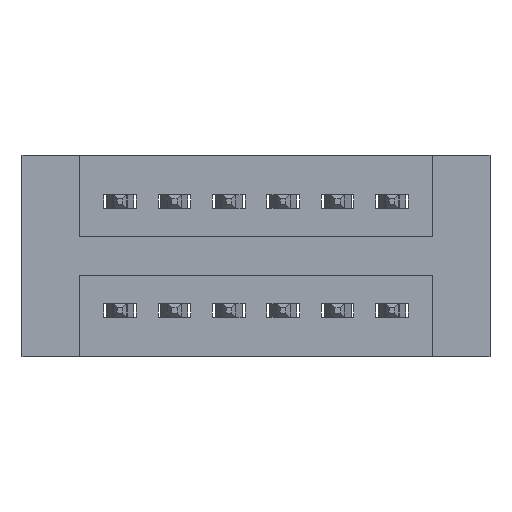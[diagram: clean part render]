
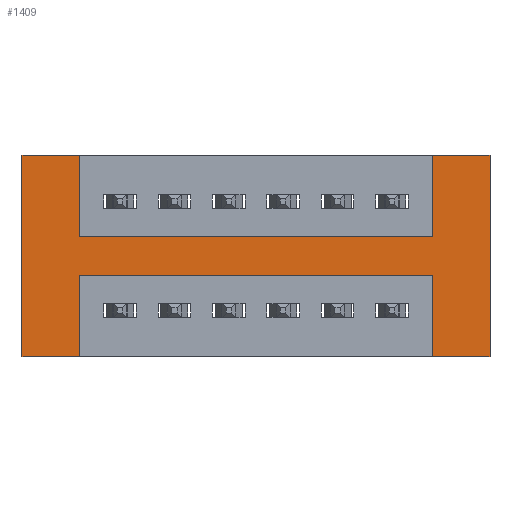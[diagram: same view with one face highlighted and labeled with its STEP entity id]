
A CAD part, front view. The second image highlights one B-rep face of the part: STEP entity #1409.
In plain terms, the highlighted planar face has unit normal (0, -1, 0).
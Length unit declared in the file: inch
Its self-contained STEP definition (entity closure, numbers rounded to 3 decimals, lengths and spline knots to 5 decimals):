
#89 = ORIENTED_EDGE ( 'NONE', *, *, #5785, .F. ) ;
#138 = CARTESIAN_POINT ( 'NONE',  ( 0.3925, 0., -0.15 ) ) ;
#204 = CARTESIAN_POINT ( 'NONE',  ( 0., 0., 0. ) ) ;
#241 = EDGE_CURVE ( 'NONE', #8746, #2887, #8727, .T. ) ;
#384 = VERTEX_POINT ( 'NONE', #6735 ) ;
#539 = VECTOR ( 'NONE', #4128, 39.37008 ) ;
#594 = VECTOR ( 'NONE', #5616, 39.37008 ) ;
#743 = PLANE ( 'NONE',  #5695 ) ;
#817 = VERTEX_POINT ( 'NONE', #7355 ) ;
#935 = EDGE_CURVE ( 'NONE', #8474, #6938, #4591, .T. ) ;
#956 = CARTESIAN_POINT ( 'NONE',  ( 0.2875, 0., 0. ) ) ;
#963 = CARTESIAN_POINT ( 'NONE',  ( 0.3925, 0., -0.15 ) ) ;
#1040 = DIRECTION ( 'NONE',  ( 0., 0., -1. ) ) ;
#1363 = VECTOR ( 'NONE', #9132, 39.37008 ) ;
#1395 = EDGE_CURVE ( 'NONE', #8628, #8474, #2612, .T. ) ;
#1409 = ADVANCED_FACE ( 'NONE', ( #6409 ), #743, .T. ) ;
#1860 = CARTESIAN_POINT ( 'NONE',  ( 0.3925, 0., 0. ) ) ;
#2245 = VERTEX_POINT ( 'NONE', #7842 ) ;
#2431 = EDGE_CURVE ( 'NONE', #5949, #2245, #8277, .T. ) ;
#2488 = LINE ( 'NONE', #2884, #6074 ) ;
#2534 = EDGE_CURVE ( 'NONE', #2245, #5627, #7633, .T. ) ;
#2536 = LINE ( 'NONE', #4183, #539 ) ;
#2612 = LINE ( 'NONE', #6999, #8086 ) ;
#2793 = VECTOR ( 'NONE', #4231, 39.37008 ) ;
#2884 = CARTESIAN_POINT ( 'NONE',  ( 0.3925, 0., -0.22 ) ) ;
#2887 = VERTEX_POINT ( 'NONE', #8492 ) ;
#2954 = CARTESIAN_POINT ( 'NONE',  ( 0.3925, 0., -0.22 ) ) ;
#3078 = LINE ( 'NONE', #4296, #6582 ) ;
#3406 = ORIENTED_EDGE ( 'NONE', *, *, #4635, .F. ) ;
#3636 = CARTESIAN_POINT ( 'NONE',  ( 1.0425, 0., -0.15 ) ) ;
#3640 = DIRECTION ( 'NONE',  ( -1., 0., 0. ) ) ;
#3722 = LINE ( 'NONE', #204, #9209 ) ;
#3738 = ORIENTED_EDGE ( 'NONE', *, *, #2534, .F. ) ;
#3787 = ORIENTED_EDGE ( 'NONE', *, *, #5757, .F. ) ;
#3859 = LINE ( 'NONE', #956, #7163 ) ;
#3908 = CARTESIAN_POINT ( 'NONE',  ( 1.0425, 0., 0. ) ) ;
#4039 = DIRECTION ( 'NONE',  ( 0., 0., 1. ) ) ;
#4128 = DIRECTION ( 'NONE',  ( 1., 0., 0. ) ) ;
#4182 = ORIENTED_EDGE ( 'NONE', *, *, #6571, .F. ) ;
#4183 = CARTESIAN_POINT ( 'NONE',  ( 0., 0., 0. ) ) ;
#4196 = CARTESIAN_POINT ( 'NONE',  ( 1.1475, 0., 0. ) ) ;
#4230 = DIRECTION ( 'NONE',  ( 0., 0., -1. ) ) ;
#4231 = DIRECTION ( 'NONE',  ( 0., 0., 1. ) ) ;
#4296 = CARTESIAN_POINT ( 'NONE',  ( 0., 0., -0.37 ) ) ;
#4338 = DIRECTION ( 'NONE',  ( -1., 0., 0. ) ) ;
#4471 = CARTESIAN_POINT ( 'NONE',  ( 0., 0., -0.37 ) ) ;
#4517 = LINE ( 'NONE', #3908, #8022 ) ;
#4591 = LINE ( 'NONE', #963, #7893 ) ;
#4635 = EDGE_CURVE ( 'NONE', #8648, #8746, #3078, .T. ) ;
#4803 = CARTESIAN_POINT ( 'NONE',  ( 0.2875, 0., -0.37 ) ) ;
#4810 = EDGE_CURVE ( 'NONE', #384, #5627, #3859, .T. ) ;
#4831 = CARTESIAN_POINT ( 'NONE',  ( 1.1475, 0., -0.37 ) ) ;
#4900 = ORIENTED_EDGE ( 'NONE', *, *, #1395, .F. ) ;
#4924 = CARTESIAN_POINT ( 'NONE',  ( 1.0425, 0., -0.37 ) ) ;
#5084 = ORIENTED_EDGE ( 'NONE', *, *, #2431, .F. ) ;
#5284 = CARTESIAN_POINT ( 'NONE',  ( 1.0425, 0., -0.37 ) ) ;
#5426 = DIRECTION ( 'NONE',  ( 1., 0., 0. ) ) ;
#5574 = ORIENTED_EDGE ( 'NONE', *, *, #8881, .F. ) ;
#5616 = DIRECTION ( 'NONE',  ( 0., 0., -1. ) ) ;
#5627 = VERTEX_POINT ( 'NONE', #4803 ) ;
#5692 = CARTESIAN_POINT ( 'NONE',  ( 1.1475, 0., 0. ) ) ;
#5695 = AXIS2_PLACEMENT_3D ( 'NONE', #4471, #7773, #4230 ) ;
#5740 = EDGE_CURVE ( 'NONE', #8648, #8075, #8226, .T. ) ;
#5757 = EDGE_CURVE ( 'NONE', #384, #8628, #2536, .T. ) ;
#5785 = EDGE_CURVE ( 'NONE', #6938, #817, #4517, .T. ) ;
#5949 = VERTEX_POINT ( 'NONE', #2954 ) ;
#6042 = DIRECTION ( 'NONE',  ( 1., 0., 0. ) ) ;
#6074 = VECTOR ( 'NONE', #3640, 39.37008 ) ;
#6409 = FACE_OUTER_BOUND ( 'NONE', #6669, .T. ) ;
#6571 = EDGE_CURVE ( 'NONE', #817, #8075, #3722, .T. ) ;
#6582 = VECTOR ( 'NONE', #4338, 39.37008 ) ;
#6647 = DIRECTION ( 'NONE',  ( -1., 0., 0. ) ) ;
#6669 = EDGE_LOOP ( 'NONE', ( #8738, #4182, #89, #8229, #4900, #3787, #6800, #3738, #5084, #5574, #6987, #3406 ) ) ;
#6678 = CARTESIAN_POINT ( 'NONE',  ( 0.3925, 0., -0.37 ) ) ;
#6687 = CARTESIAN_POINT ( 'NONE',  ( 0., 0., -0.37 ) ) ;
#6735 = CARTESIAN_POINT ( 'NONE',  ( 0.2875, 0., 0. ) ) ;
#6800 = ORIENTED_EDGE ( 'NONE', *, *, #4810, .T. ) ;
#6896 = DIRECTION ( 'NONE',  ( 0., 0., -1. ) ) ;
#6938 = VERTEX_POINT ( 'NONE', #3636 ) ;
#6987 = ORIENTED_EDGE ( 'NONE', *, *, #241, .F. ) ;
#6999 = CARTESIAN_POINT ( 'NONE',  ( 0.3925, 0., 0. ) ) ;
#7163 = VECTOR ( 'NONE', #1040, 39.37008 ) ;
#7355 = CARTESIAN_POINT ( 'NONE',  ( 1.0425, 0., 0. ) ) ;
#7413 = VECTOR ( 'NONE', #6647, 39.37008 ) ;
#7633 = LINE ( 'NONE', #6687, #7413 ) ;
#7773 = DIRECTION ( 'NONE',  ( 0., -1., 0. ) ) ;
#7842 = CARTESIAN_POINT ( 'NONE',  ( 0.3925, 0., -0.37 ) ) ;
#7893 = VECTOR ( 'NONE', #6042, 39.37008 ) ;
#8022 = VECTOR ( 'NONE', #4039, 39.37008 ) ;
#8075 = VERTEX_POINT ( 'NONE', #5692 ) ;
#8086 = VECTOR ( 'NONE', #6896, 39.37008 ) ;
#8226 = LINE ( 'NONE', #4196, #2793 ) ;
#8229 = ORIENTED_EDGE ( 'NONE', *, *, #935, .F. ) ;
#8277 = LINE ( 'NONE', #6678, #594 ) ;
#8474 = VERTEX_POINT ( 'NONE', #138 ) ;
#8492 = CARTESIAN_POINT ( 'NONE',  ( 1.0425, 0., -0.22 ) ) ;
#8628 = VERTEX_POINT ( 'NONE', #1860 ) ;
#8648 = VERTEX_POINT ( 'NONE', #4831 ) ;
#8727 = LINE ( 'NONE', #5284, #1363 ) ;
#8738 = ORIENTED_EDGE ( 'NONE', *, *, #5740, .T. ) ;
#8746 = VERTEX_POINT ( 'NONE', #4924 ) ;
#8881 = EDGE_CURVE ( 'NONE', #2887, #5949, #2488, .T. ) ;
#9132 = DIRECTION ( 'NONE',  ( 0., 0., 1. ) ) ;
#9209 = VECTOR ( 'NONE', #5426, 39.37008 ) ;
